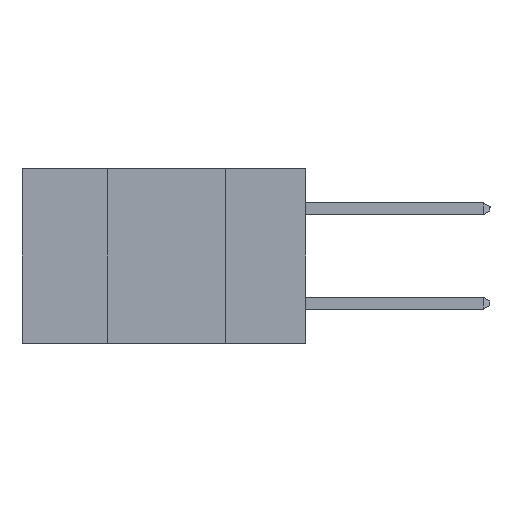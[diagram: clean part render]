
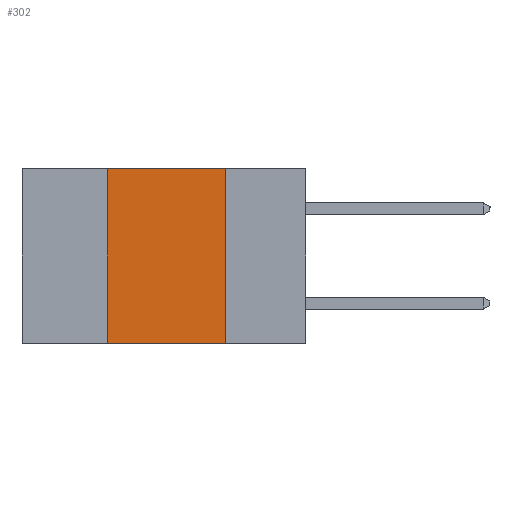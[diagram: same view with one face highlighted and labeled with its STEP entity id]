
A CAD part, left-side view. The second image highlights one B-rep face of the part: STEP entity #302.
In plain terms, the highlighted planar face has unit normal (-1, 0, 0).
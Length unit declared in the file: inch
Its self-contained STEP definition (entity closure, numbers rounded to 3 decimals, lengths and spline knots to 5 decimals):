
#302 = ADVANCED_FACE ( 'NONE', ( #4149 ), #7818, .F. ) ;
#449 = VERTEX_POINT ( 'NONE', #8959 ) ;
#537 = DIRECTION ( 'NONE',  ( 0., 0., -1. ) ) ;
#669 = ORIENTED_EDGE ( 'NONE', *, *, #5880, .T. ) ;
#784 = LINE ( 'NONE', #10286, #10171 ) ;
#1513 = ORIENTED_EDGE ( 'NONE', *, *, #1807, .F. ) ;
#1647 = DIRECTION ( 'NONE',  ( 0., 0., 1. ) ) ;
#1766 = CARTESIAN_POINT ( 'NONE',  ( 0., 0.42, 0. ) ) ;
#1807 = EDGE_CURVE ( 'NONE', #2883, #4323, #10785, .T. ) ;
#2389 = ORIENTED_EDGE ( 'NONE', *, *, #9540, .F. ) ;
#2595 = DIRECTION ( 'NONE',  ( 0., -1., 0. ) ) ;
#2883 = VERTEX_POINT ( 'NONE', #6578 ) ;
#3560 = EDGE_LOOP ( 'NONE', ( #11165, #2389, #1513, #669 ) ) ;
#3900 = VECTOR ( 'NONE', #2595, 39.37008 ) ;
#4149 = FACE_OUTER_BOUND ( 'NONE', #3560, .T. ) ;
#4268 = CARTESIAN_POINT ( 'NONE',  ( 0., 0.6, 0. ) ) ;
#4323 = VERTEX_POINT ( 'NONE', #1766 ) ;
#4847 = CARTESIAN_POINT ( 'NONE',  ( 0., 0.17, -0.37 ) ) ;
#5277 = VECTOR ( 'NONE', #537, 39.37008 ) ;
#5880 = EDGE_CURVE ( 'NONE', #2883, #9105, #784, .T. ) ;
#6492 = CARTESIAN_POINT ( 'NONE',  ( 0., 0.42, -0.37 ) ) ;
#6578 = CARTESIAN_POINT ( 'NONE',  ( 0., 0.42, -0.37 ) ) ;
#6812 = DIRECTION ( 'NONE',  ( 0., -1., 0. ) ) ;
#6885 = CARTESIAN_POINT ( 'NONE',  ( 0., 0.6, 0. ) ) ;
#7008 = CARTESIAN_POINT ( 'NONE',  ( 0., 0.17, -0.37 ) ) ;
#7717 = DIRECTION ( 'NONE',  ( 1., 0., 0. ) ) ;
#7818 = PLANE ( 'NONE',  #7845 ) ;
#7845 = AXIS2_PLACEMENT_3D ( 'NONE', #4268, #7717, #8738 ) ;
#8738 = DIRECTION ( 'NONE',  ( 0., 0., -1. ) ) ;
#8822 = VECTOR ( 'NONE', #1647, 39.37008 ) ;
#8959 = CARTESIAN_POINT ( 'NONE',  ( 0., 0.17, 0. ) ) ;
#9105 = VERTEX_POINT ( 'NONE', #7008 ) ;
#9540 = EDGE_CURVE ( 'NONE', #4323, #449, #11316, .T. ) ;
#10139 = LINE ( 'NONE', #4847, #5277 ) ;
#10171 = VECTOR ( 'NONE', #6812, 39.37008 ) ;
#10272 = EDGE_CURVE ( 'NONE', #449, #9105, #10139, .T. ) ;
#10286 = CARTESIAN_POINT ( 'NONE',  ( 0., 0.6, -0.37 ) ) ;
#10785 = LINE ( 'NONE', #6492, #8822 ) ;
#11165 = ORIENTED_EDGE ( 'NONE', *, *, #10272, .F. ) ;
#11316 = LINE ( 'NONE', #6885, #3900 ) ;
